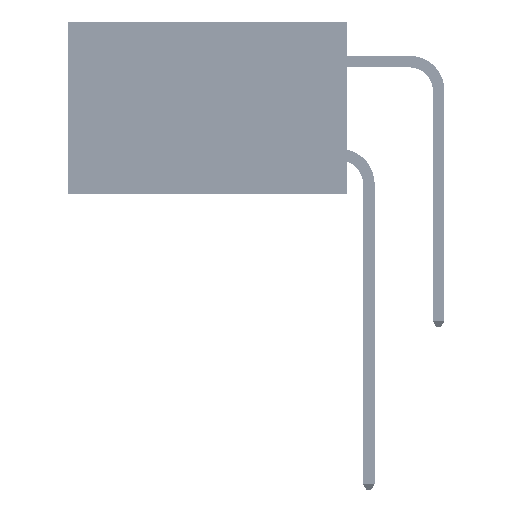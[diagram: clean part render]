
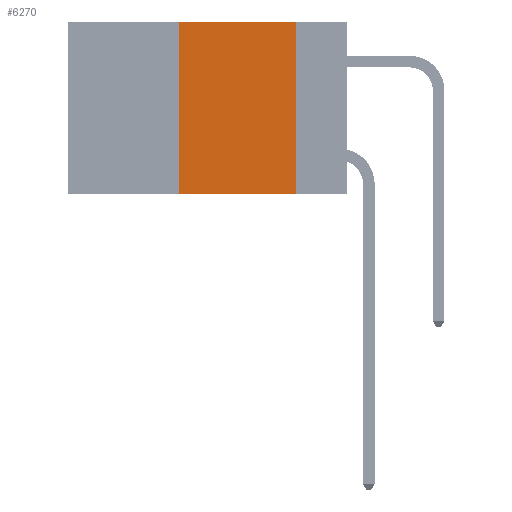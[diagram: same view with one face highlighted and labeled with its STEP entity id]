
A CAD part, left-side view. The second image highlights one B-rep face of the part: STEP entity #6270.
In plain terms, the highlighted planar face has unit normal (-1, 0, 0).
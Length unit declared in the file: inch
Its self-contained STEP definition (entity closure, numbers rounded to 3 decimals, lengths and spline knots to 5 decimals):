
#264 = AXIS2_PLACEMENT_3D ( 'NONE', #24059, #38760, #27544 ) ;
#2448 = ORIENTED_EDGE ( 'NONE', *, *, #19308, .F. ) ;
#2641 = VECTOR ( 'NONE', #11986, 39.37008 ) ;
#2643 = ORIENTED_EDGE ( 'NONE', *, *, #5714, .T. ) ;
#3470 = EDGE_CURVE ( 'NONE', #20557, #38979, #25688, .T. ) ;
#4593 = VECTOR ( 'NONE', #25331, 39.37008 ) ;
#5714 = EDGE_CURVE ( 'NONE', #39903, #38979, #29084, .T. ) ;
#6270 = ADVANCED_FACE ( 'NONE', ( #28987 ), #12323, .F. ) ;
#11986 = DIRECTION ( 'NONE',  ( 0., 0., -1. ) ) ;
#12323 = PLANE ( 'NONE',  #264 ) ;
#13769 = CARTESIAN_POINT ( 'NONE',  ( 0., 0.6, 0. ) ) ;
#16784 = ORIENTED_EDGE ( 'NONE', *, *, #3470, .F. ) ;
#17181 = CARTESIAN_POINT ( 'NONE',  ( 0., 0.11, 0. ) ) ;
#18756 = DIRECTION ( 'NONE',  ( 0., 0., 1. ) ) ;
#19088 = VECTOR ( 'NONE', #39137, 39.37008 ) ;
#19308 = EDGE_CURVE ( 'NONE', #39903, #32843, #45299, .T. ) ;
#20557 = VERTEX_POINT ( 'NONE', #17181 ) ;
#20901 = CARTESIAN_POINT ( 'NONE',  ( 0., 0.36, 0. ) ) ;
#22983 = EDGE_CURVE ( 'NONE', #32843, #20557, #40674, .T. ) ;
#24059 = CARTESIAN_POINT ( 'NONE',  ( 0., 0.6, 0. ) ) ;
#24144 = CARTESIAN_POINT ( 'NONE',  ( 0., 0.11, -0.37 ) ) ;
#25331 = DIRECTION ( 'NONE',  ( 0., -1., 0. ) ) ;
#25688 = LINE ( 'NONE', #34470, #2641 ) ;
#26930 = VECTOR ( 'NONE', #18756, 39.37008 ) ;
#27544 = DIRECTION ( 'NONE',  ( 0., 0., -1. ) ) ;
#28987 = FACE_OUTER_BOUND ( 'NONE', #31416, .T. ) ;
#28994 = CARTESIAN_POINT ( 'NONE',  ( 0., 0.36, -0.37 ) ) ;
#29084 = LINE ( 'NONE', #35822, #19088 ) ;
#31416 = EDGE_LOOP ( 'NONE', ( #16784, #34930, #2448, #2643 ) ) ;
#32843 = VERTEX_POINT ( 'NONE', #20901 ) ;
#34470 = CARTESIAN_POINT ( 'NONE',  ( 0., 0.11, 0. ) ) ;
#34930 = ORIENTED_EDGE ( 'NONE', *, *, #22983, .F. ) ;
#35822 = CARTESIAN_POINT ( 'NONE',  ( 0., 0.6, -0.37 ) ) ;
#38760 = DIRECTION ( 'NONE',  ( 1., 0., 0. ) ) ;
#38979 = VERTEX_POINT ( 'NONE', #24144 ) ;
#39137 = DIRECTION ( 'NONE',  ( 0., -1., 0. ) ) ;
#39903 = VERTEX_POINT ( 'NONE', #28994 ) ;
#40674 = LINE ( 'NONE', #13769, #4593 ) ;
#41034 = CARTESIAN_POINT ( 'NONE',  ( 0., 0.36, 0. ) ) ;
#45299 = LINE ( 'NONE', #41034, #26930 ) ;
